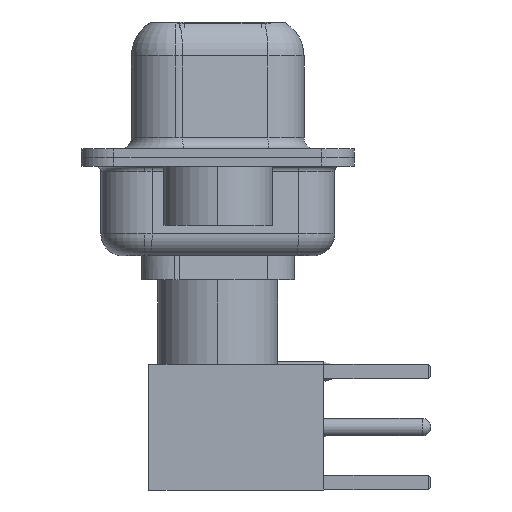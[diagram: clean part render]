
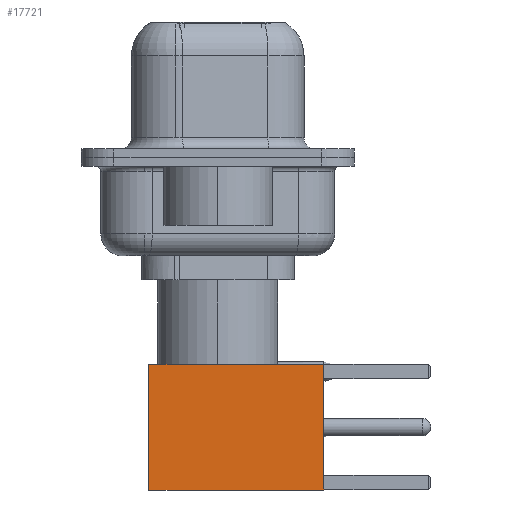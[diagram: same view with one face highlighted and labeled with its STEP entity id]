
A CAD part, left-side view. The second image highlights one B-rep face of the part: STEP entity #17721.
In plain terms, the highlighted face is planar.
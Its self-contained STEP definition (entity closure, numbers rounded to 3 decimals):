
#534 = CARTESIAN_POINT ( 'NONE',  ( 0., 2.875, 8. ) ) ;
#2170 = LINE ( 'NONE', #20003, #22634 ) ;
#3327 = CARTESIAN_POINT ( 'NONE',  ( 2.875, 2.875, 0. ) ) ;
#3553 = CARTESIAN_POINT ( 'NONE',  ( -2.875, 2.875, 0. ) ) ;
#4316 = DIRECTION ( 'NONE',  ( -1., 0., 0. ) ) ;
#4593 = LINE ( 'NONE', #534, #7202 ) ;
#5289 = AXIS2_PLACEMENT_3D ( 'NONE', #18389, #8395, #18634 ) ;
#5482 = VERTEX_POINT ( 'NONE', #23837 ) ;
#6554 = EDGE_CURVE ( 'NONE', #5482, #21254, #4593, .T. ) ;
#6568 = FACE_OUTER_BOUND ( 'NONE', #16773, .T. ) ;
#6690 = DIRECTION ( 'NONE',  ( -1., 0., 0. ) ) ;
#7202 = VECTOR ( 'NONE', #6690, 1000. ) ;
#7942 = CARTESIAN_POINT ( 'NONE',  ( -2.875, 2.875, 0. ) ) ;
#8250 = LINE ( 'NONE', #16248, #19987 ) ;
#8395 = DIRECTION ( 'NONE',  ( 0., 1., 0. ) ) ;
#8963 = VERTEX_POINT ( 'NONE', #7942 ) ;
#10131 = ORIENTED_EDGE ( 'NONE', *, *, #20442, .F. ) ;
#10720 = EDGE_CURVE ( 'NONE', #5482, #13518, #2170, .T. ) ;
#12113 = VECTOR ( 'NONE', #21540, 1000. ) ;
#12285 = ORIENTED_EDGE ( 'NONE', *, *, #10720, .T. ) ;
#12472 = PLANE ( 'NONE',  #5289 ) ;
#13518 = VERTEX_POINT ( 'NONE', #3327 ) ;
#14558 = CARTESIAN_POINT ( 'NONE',  ( -2.875, 2.875, 8. ) ) ;
#16248 = CARTESIAN_POINT ( 'NONE',  ( 0., 2.875, 0. ) ) ;
#16773 = EDGE_LOOP ( 'NONE', ( #12285, #25215, #10131, #19064 ) ) ;
#17721 = ADVANCED_FACE ( 'NONE', ( #6568 ), #12472, .T. ) ;
#18252 = EDGE_CURVE ( 'NONE', #13518, #8963, #8250, .T. ) ;
#18389 = CARTESIAN_POINT ( 'NONE',  ( 2.875, 2.875, 0. ) ) ;
#18634 = DIRECTION ( 'NONE',  ( 0., 0., 1. ) ) ;
#19064 = ORIENTED_EDGE ( 'NONE', *, *, #6554, .F. ) ;
#19987 = VECTOR ( 'NONE', #4316, 1000. ) ;
#20003 = CARTESIAN_POINT ( 'NONE',  ( 2.875, 2.875, 0. ) ) ;
#20390 = DIRECTION ( 'NONE',  ( 0., 0., -1. ) ) ;
#20442 = EDGE_CURVE ( 'NONE', #21254, #8963, #25594, .T. ) ;
#21254 = VERTEX_POINT ( 'NONE', #14558 ) ;
#21540 = DIRECTION ( 'NONE',  ( 0., 0., -1. ) ) ;
#22634 = VECTOR ( 'NONE', #20390, 1000. ) ;
#23837 = CARTESIAN_POINT ( 'NONE',  ( 2.875, 2.875, 8. ) ) ;
#25215 = ORIENTED_EDGE ( 'NONE', *, *, #18252, .T. ) ;
#25594 = LINE ( 'NONE', #3553, #12113 ) ;
